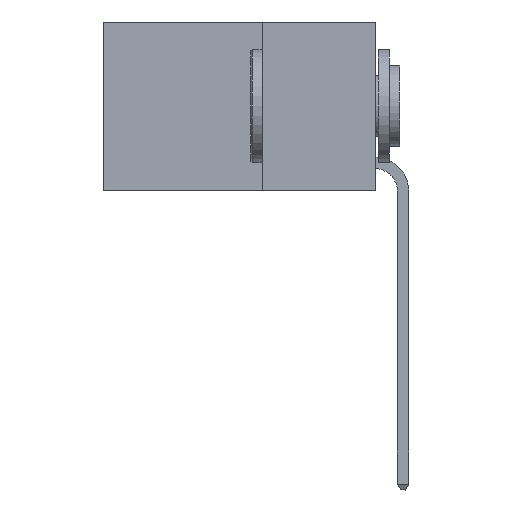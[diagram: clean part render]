
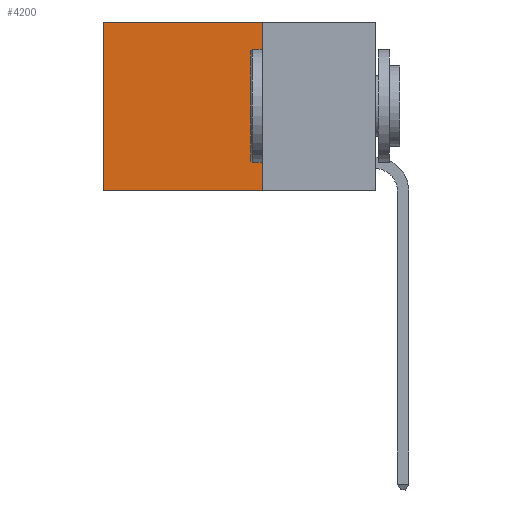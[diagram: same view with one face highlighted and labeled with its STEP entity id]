
A CAD part, left-side view. The second image highlights one B-rep face of the part: STEP entity #4200.
In plain terms, the highlighted planar face has unit normal (-1, 0, 0).
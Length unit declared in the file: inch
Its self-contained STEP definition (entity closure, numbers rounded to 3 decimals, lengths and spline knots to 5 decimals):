
#36 = FACE_OUTER_BOUND ( 'NONE', #2105, .T. ) ;
#799 = ORIENTED_EDGE ( 'NONE', *, *, #21830, .T. ) ;
#951 = VECTOR ( 'NONE', #11365, 39.37008 ) ;
#1531 = VECTOR ( 'NONE', #10135, 39.37008 ) ;
#1935 = DIRECTION ( 'NONE',  ( 0., 0., -1. ) ) ;
#2105 = EDGE_LOOP ( 'NONE', ( #6768, #16435, #12081, #799 ) ) ;
#2207 = LINE ( 'NONE', #8120, #1531 ) ;
#2262 = DIRECTION ( 'NONE',  ( 1., 0., 0. ) ) ;
#2468 = VECTOR ( 'NONE', #1935, 39.37008 ) ;
#4200 = ADVANCED_FACE ( 'NONE', ( #36 ), #14548, .F. ) ;
#4774 = EDGE_CURVE ( 'NONE', #10748, #21119, #18658, .T. ) ;
#4890 = VERTEX_POINT ( 'NONE', #20574 ) ;
#5771 = EDGE_CURVE ( 'NONE', #21119, #4890, #12026, .T. ) ;
#6768 = ORIENTED_EDGE ( 'NONE', *, *, #14238, .T. ) ;
#6868 = VERTEX_POINT ( 'NONE', #23684 ) ;
#8120 = CARTESIAN_POINT ( 'NONE',  ( 0.2625, 0.25, 0. ) ) ;
#10135 = DIRECTION ( 'NONE',  ( 0., 1., 0. ) ) ;
#10258 = CARTESIAN_POINT ( 'NONE',  ( 0.2625, 0.25, 0. ) ) ;
#10554 = CARTESIAN_POINT ( 'NONE',  ( 0.2625, 0.25, 0. ) ) ;
#10748 = VERTEX_POINT ( 'NONE', #17922 ) ;
#11365 = DIRECTION ( 'NONE',  ( 0., 1., 0. ) ) ;
#12026 = LINE ( 'NONE', #25270, #951 ) ;
#12081 = ORIENTED_EDGE ( 'NONE', *, *, #4774, .F. ) ;
#12702 = VECTOR ( 'NONE', #16291, 39.37008 ) ;
#13415 = LINE ( 'NONE', #26153, #2468 ) ;
#14238 = EDGE_CURVE ( 'NONE', #6868, #4890, #13415, .T. ) ;
#14548 = PLANE ( 'NONE',  #14560 ) ;
#14560 = AXIS2_PLACEMENT_3D ( 'NONE', #10554, #2262, #16583 ) ;
#16291 = DIRECTION ( 'NONE',  ( 0., 0., -1. ) ) ;
#16435 = ORIENTED_EDGE ( 'NONE', *, *, #5771, .F. ) ;
#16583 = DIRECTION ( 'NONE',  ( 0., 0., -1. ) ) ;
#17922 = CARTESIAN_POINT ( 'NONE',  ( 0.2625, 0.25, 0. ) ) ;
#18658 = LINE ( 'NONE', #10258, #12702 ) ;
#19721 = CARTESIAN_POINT ( 'NONE',  ( 0.2625, 0.25, -0.37 ) ) ;
#20574 = CARTESIAN_POINT ( 'NONE',  ( 0.2625, 0.6, -0.37 ) ) ;
#21119 = VERTEX_POINT ( 'NONE', #19721 ) ;
#21830 = EDGE_CURVE ( 'NONE', #10748, #6868, #2207, .T. ) ;
#23684 = CARTESIAN_POINT ( 'NONE',  ( 0.2625, 0.6, 0. ) ) ;
#25270 = CARTESIAN_POINT ( 'NONE',  ( 0.2625, 0.25, -0.37 ) ) ;
#26153 = CARTESIAN_POINT ( 'NONE',  ( 0.2625, 0.6, 0. ) ) ;
